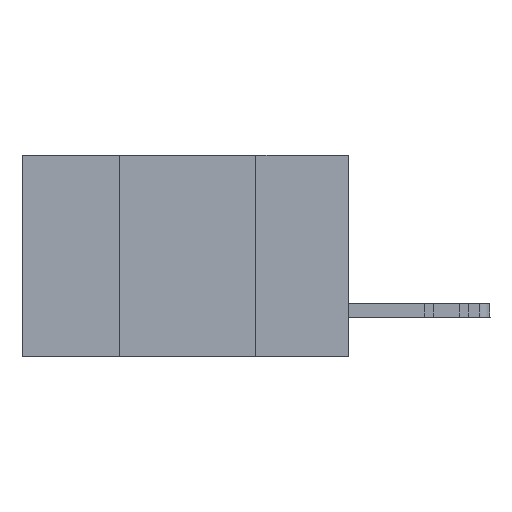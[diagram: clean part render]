
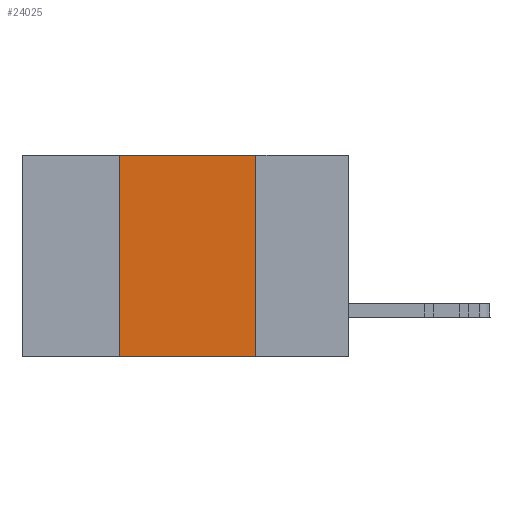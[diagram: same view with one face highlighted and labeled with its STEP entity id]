
A CAD part, left-side view. The second image highlights one B-rep face of the part: STEP entity #24025.
In plain terms, the highlighted planar face has unit normal (-1, 0, 0).
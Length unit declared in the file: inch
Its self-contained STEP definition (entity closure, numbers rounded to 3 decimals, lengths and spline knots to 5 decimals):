
#11 = EDGE_LOOP ( 'NONE', ( #26647, #15544, #3661, #28482 ) ) ;
#919 = VECTOR ( 'NONE', #16572, 39.37008 ) ;
#2072 = DIRECTION ( 'NONE',  ( 0., -1., 0. ) ) ;
#3238 = DIRECTION ( 'NONE',  ( 0., 0., 1. ) ) ;
#3661 = ORIENTED_EDGE ( 'NONE', *, *, #4175, .F. ) ;
#4074 = LINE ( 'NONE', #28579, #919 ) ;
#4175 = EDGE_CURVE ( 'NONE', #8667, #15963, #24938, .T. ) ;
#5159 = CARTESIAN_POINT ( 'NONE',  ( 0., 0.42, 0. ) ) ;
#5659 = VERTEX_POINT ( 'NONE', #23168 ) ;
#5963 = AXIS2_PLACEMENT_3D ( 'NONE', #9123, #30489, #25759 ) ;
#6227 = VERTEX_POINT ( 'NONE', #23584 ) ;
#6250 = EDGE_CURVE ( 'NONE', #15963, #6227, #7149, .T. ) ;
#7149 = LINE ( 'NONE', #26299, #22781 ) ;
#7789 = VECTOR ( 'NONE', #17828, 39.37008 ) ;
#8667 = VERTEX_POINT ( 'NONE', #24132 ) ;
#9123 = CARTESIAN_POINT ( 'NONE',  ( 0., 0.6, 0. ) ) ;
#10706 = CARTESIAN_POINT ( 'NONE',  ( 0., 0.6, -0.37 ) ) ;
#15544 = ORIENTED_EDGE ( 'NONE', *, *, #6250, .F. ) ;
#15963 = VERTEX_POINT ( 'NONE', #18537 ) ;
#16186 = EDGE_CURVE ( 'NONE', #6227, #5659, #4074, .T. ) ;
#16567 = FACE_OUTER_BOUND ( 'NONE', #11, .T. ) ;
#16572 = DIRECTION ( 'NONE',  ( 0., 0., -1. ) ) ;
#17828 = DIRECTION ( 'NONE',  ( 0., -1., 0. ) ) ;
#17976 = LINE ( 'NONE', #10706, #7789 ) ;
#18421 = EDGE_CURVE ( 'NONE', #8667, #5659, #17976, .T. ) ;
#18537 = CARTESIAN_POINT ( 'NONE',  ( 0., 0.42, 0. ) ) ;
#20839 = PLANE ( 'NONE',  #5963 ) ;
#22781 = VECTOR ( 'NONE', #2072, 39.37008 ) ;
#23168 = CARTESIAN_POINT ( 'NONE',  ( 0., 0.17, -0.37 ) ) ;
#23584 = CARTESIAN_POINT ( 'NONE',  ( 0., 0.17, 0. ) ) ;
#24025 = ADVANCED_FACE ( 'NONE', ( #16567 ), #20839, .F. ) ;
#24132 = CARTESIAN_POINT ( 'NONE',  ( 0., 0.42, -0.37 ) ) ;
#24938 = LINE ( 'NONE', #5159, #27258 ) ;
#25759 = DIRECTION ( 'NONE',  ( 0., 0., -1. ) ) ;
#26299 = CARTESIAN_POINT ( 'NONE',  ( 0., 0.6, 0. ) ) ;
#26647 = ORIENTED_EDGE ( 'NONE', *, *, #16186, .F. ) ;
#27258 = VECTOR ( 'NONE', #3238, 39.37008 ) ;
#28482 = ORIENTED_EDGE ( 'NONE', *, *, #18421, .T. ) ;
#28579 = CARTESIAN_POINT ( 'NONE',  ( 0., 0.17, 0. ) ) ;
#30489 = DIRECTION ( 'NONE',  ( 1., 0., 0. ) ) ;
